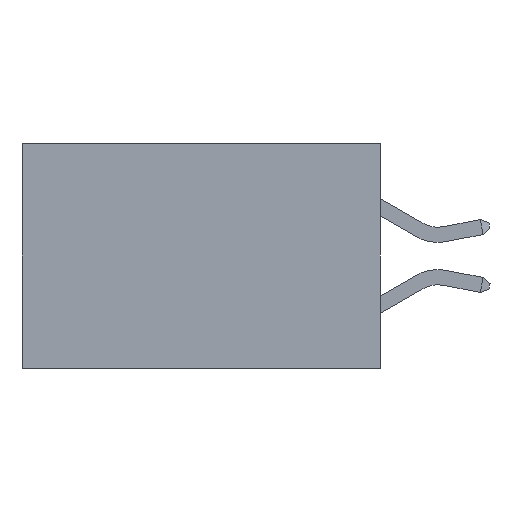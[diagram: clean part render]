
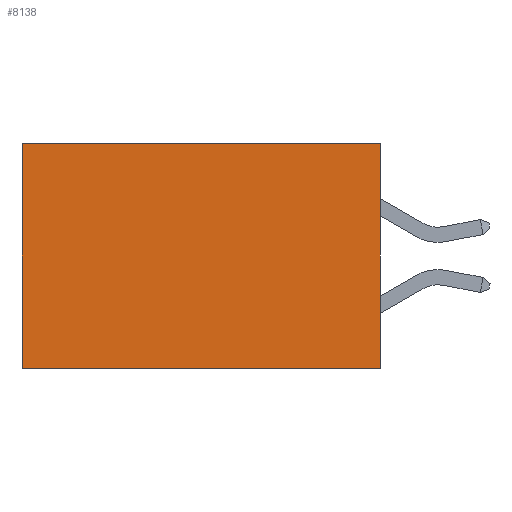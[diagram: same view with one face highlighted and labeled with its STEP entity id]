
A CAD part, left-side view. The second image highlights one B-rep face of the part: STEP entity #8138.
In plain terms, the highlighted planar face has unit normal (-1, 0, 0).
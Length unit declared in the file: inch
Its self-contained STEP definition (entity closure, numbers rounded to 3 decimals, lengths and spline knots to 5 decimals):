
#3 = ORIENTED_EDGE ( 'NONE', *, *, #5260, .F. ) ;
#112 = DIRECTION ( 'NONE',  ( 0., 1., 0. ) ) ;
#136 = AXIS2_PLACEMENT_3D ( 'NONE', #2785, #11896, #6615 ) ;
#501 = LINE ( 'NONE', #9980, #10076 ) ;
#1205 = CARTESIAN_POINT ( 'NONE',  ( 0.277, 0., 0. ) ) ;
#1447 = LINE ( 'NONE', #2116, #3697 ) ;
#1646 = LINE ( 'NONE', #8591, #8572 ) ;
#2116 = CARTESIAN_POINT ( 'NONE',  ( 0.277, 0., -0.37 ) ) ;
#2785 = CARTESIAN_POINT ( 'NONE',  ( 0.277, 0., -0.37 ) ) ;
#2935 = CARTESIAN_POINT ( 'NONE',  ( 0.277, 0., -0.37 ) ) ;
#3341 = ORIENTED_EDGE ( 'NONE', *, *, #10085, .T. ) ;
#3527 = VERTEX_POINT ( 'NONE', #1205 ) ;
#3537 = DIRECTION ( 'NONE',  ( 0., 0., -1. ) ) ;
#3697 = VECTOR ( 'NONE', #6674, 39.37008 ) ;
#3954 = VERTEX_POINT ( 'NONE', #7976 ) ;
#4328 = CARTESIAN_POINT ( 'NONE',  ( 0.277, 0., -0.37 ) ) ;
#4819 = EDGE_LOOP ( 'NONE', ( #3341, #3, #9073, #10045 ) ) ;
#5260 = EDGE_CURVE ( 'NONE', #5294, #11746, #1447, .T. ) ;
#5294 = VERTEX_POINT ( 'NONE', #4328 ) ;
#5876 = LINE ( 'NONE', #2935, #10059 ) ;
#6615 = DIRECTION ( 'NONE',  ( 0., 0., -1. ) ) ;
#6674 = DIRECTION ( 'NONE',  ( 0., 1., 0. ) ) ;
#7976 = CARTESIAN_POINT ( 'NONE',  ( 0.277, 0.59, 0. ) ) ;
#8138 = ADVANCED_FACE ( 'NONE', ( #8716 ), #11000, .F. ) ;
#8542 = DIRECTION ( 'NONE',  ( 0., 0., -1. ) ) ;
#8572 = VECTOR ( 'NONE', #112, 39.37008 ) ;
#8591 = CARTESIAN_POINT ( 'NONE',  ( 0.277, 0., 0. ) ) ;
#8716 = FACE_OUTER_BOUND ( 'NONE', #4819, .T. ) ;
#8812 = EDGE_CURVE ( 'NONE', #3527, #3954, #1646, .T. ) ;
#9073 = ORIENTED_EDGE ( 'NONE', *, *, #10927, .F. ) ;
#9611 = CARTESIAN_POINT ( 'NONE',  ( 0.277, 0.59, -0.37 ) ) ;
#9980 = CARTESIAN_POINT ( 'NONE',  ( 0.277, 0.59, -0.37 ) ) ;
#10045 = ORIENTED_EDGE ( 'NONE', *, *, #8812, .T. ) ;
#10059 = VECTOR ( 'NONE', #8542, 39.37008 ) ;
#10076 = VECTOR ( 'NONE', #3537, 39.37008 ) ;
#10085 = EDGE_CURVE ( 'NONE', #3954, #11746, #501, .T. ) ;
#10927 = EDGE_CURVE ( 'NONE', #3527, #5294, #5876, .T. ) ;
#11000 = PLANE ( 'NONE',  #136 ) ;
#11746 = VERTEX_POINT ( 'NONE', #9611 ) ;
#11896 = DIRECTION ( 'NONE',  ( 1., 0., 0. ) ) ;
